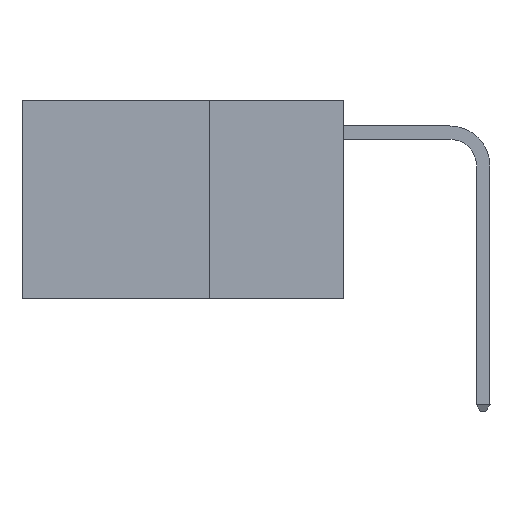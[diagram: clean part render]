
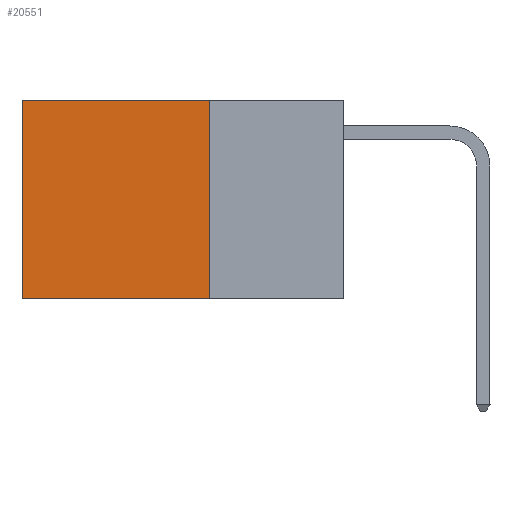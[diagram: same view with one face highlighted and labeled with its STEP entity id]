
A CAD part, left-side view. The second image highlights one B-rep face of the part: STEP entity #20551.
In plain terms, the highlighted planar face has unit normal (-1, 0, 0).
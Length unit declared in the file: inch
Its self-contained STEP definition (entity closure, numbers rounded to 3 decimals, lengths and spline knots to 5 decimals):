
#491 = LINE ( 'NONE', #20865, #24159 ) ;
#637 = DIRECTION ( 'NONE',  ( 0., 1., 0. ) ) ;
#745 = VECTOR ( 'NONE', #10920, 39.37008 ) ;
#855 = PLANE ( 'NONE',  #10464 ) ;
#1323 = LINE ( 'NONE', #1828, #10831 ) ;
#1828 = CARTESIAN_POINT ( 'NONE',  ( 0.2625, 0.25, 0. ) ) ;
#1957 = LINE ( 'NONE', #14584, #745 ) ;
#2854 = DIRECTION ( 'NONE',  ( 1., 0., 0. ) ) ;
#3013 = VECTOR ( 'NONE', #637, 39.37008 ) ;
#5909 = ORIENTED_EDGE ( 'NONE', *, *, #12301, .F. ) ;
#6486 = CARTESIAN_POINT ( 'NONE',  ( 0.2625, 0.6, -0.37 ) ) ;
#8032 = EDGE_CURVE ( 'NONE', #21779, #13000, #1957, .T. ) ;
#8511 = VERTEX_POINT ( 'NONE', #23232 ) ;
#8534 = CARTESIAN_POINT ( 'NONE',  ( 0.2625, 0.25, 0. ) ) ;
#10156 = VERTEX_POINT ( 'NONE', #18012 ) ;
#10464 = AXIS2_PLACEMENT_3D ( 'NONE', #8534, #2854, #16046 ) ;
#10831 = VECTOR ( 'NONE', #11317, 39.37008 ) ;
#10920 = DIRECTION ( 'NONE',  ( 0., 0., -1. ) ) ;
#11317 = DIRECTION ( 'NONE',  ( 0., 1., 0. ) ) ;
#12301 = EDGE_CURVE ( 'NONE', #10156, #13000, #17457, .T. ) ;
#13000 = VERTEX_POINT ( 'NONE', #6486 ) ;
#13576 = DIRECTION ( 'NONE',  ( 0., 0., -1. ) ) ;
#13857 = FACE_OUTER_BOUND ( 'NONE', #16132, .T. ) ;
#14584 = CARTESIAN_POINT ( 'NONE',  ( 0.2625, 0.6, 0. ) ) ;
#14990 = EDGE_CURVE ( 'NONE', #8511, #10156, #491, .T. ) ;
#15336 = ORIENTED_EDGE ( 'NONE', *, *, #14990, .F. ) ;
#16046 = DIRECTION ( 'NONE',  ( 0., 0., -1. ) ) ;
#16132 = EDGE_LOOP ( 'NONE', ( #16331, #5909, #15336, #22494 ) ) ;
#16331 = ORIENTED_EDGE ( 'NONE', *, *, #8032, .T. ) ;
#16748 = EDGE_CURVE ( 'NONE', #8511, #21779, #1323, .T. ) ;
#17457 = LINE ( 'NONE', #17639, #3013 ) ;
#17639 = CARTESIAN_POINT ( 'NONE',  ( 0.2625, 0.25, -0.37 ) ) ;
#18012 = CARTESIAN_POINT ( 'NONE',  ( 0.2625, 0.25, -0.37 ) ) ;
#20551 = ADVANCED_FACE ( 'NONE', ( #13857 ), #855, .F. ) ;
#20865 = CARTESIAN_POINT ( 'NONE',  ( 0.2625, 0.25, 0. ) ) ;
#21779 = VERTEX_POINT ( 'NONE', #23419 ) ;
#22494 = ORIENTED_EDGE ( 'NONE', *, *, #16748, .T. ) ;
#23232 = CARTESIAN_POINT ( 'NONE',  ( 0.2625, 0.25, 0. ) ) ;
#23419 = CARTESIAN_POINT ( 'NONE',  ( 0.2625, 0.6, 0. ) ) ;
#24159 = VECTOR ( 'NONE', #13576, 39.37008 ) ;
